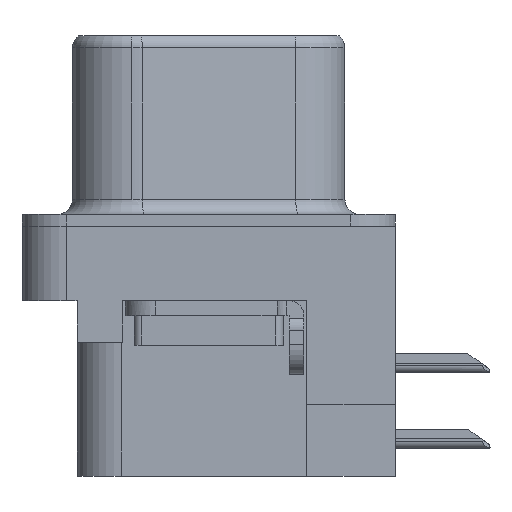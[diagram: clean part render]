
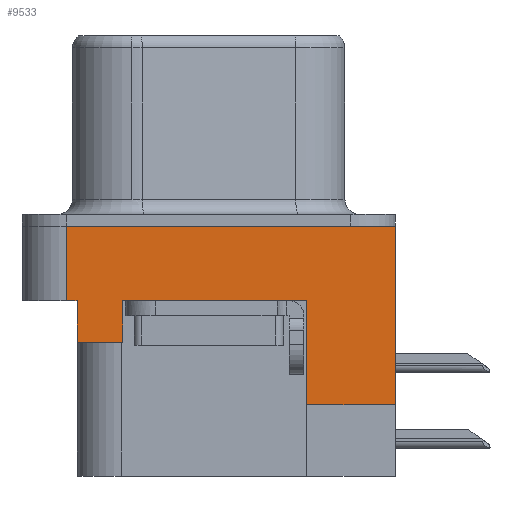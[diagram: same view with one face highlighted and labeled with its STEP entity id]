
A CAD part, left-side view. The second image highlights one B-rep face of the part: STEP entity #9533.
In plain terms, the highlighted planar face has unit normal (-1, 0, 0).
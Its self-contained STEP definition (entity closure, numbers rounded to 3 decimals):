
#211 = ORIENTED_EDGE ( 'NONE', *, *, #20539, .F. ) ;
#467 = VERTEX_POINT ( 'NONE', #12002 ) ;
#637 = VECTOR ( 'NONE', #18325, 1000. ) ;
#644 = CARTESIAN_POINT ( 'NONE',  ( -3., 2.895, -3.9 ) ) ;
#812 = LINE ( 'NONE', #14703, #637 ) ;
#1018 = DIRECTION ( 'NONE',  ( 0., 1., 0. ) ) ;
#1328 = AXIS2_PLACEMENT_3D ( 'NONE', #19992, #2776, #14723 ) ;
#1595 = ORIENTED_EDGE ( 'NONE', *, *, #21000, .T. ) ;
#1665 = DIRECTION ( 'NONE',  ( 0., 0., 1. ) ) ;
#2381 = VERTEX_POINT ( 'NONE', #3342 ) ;
#2776 = DIRECTION ( 'NONE',  ( -1., 0., 0. ) ) ;
#3298 = CARTESIAN_POINT ( 'NONE',  ( -3., 4.425, -3.9 ) ) ;
#3342 = CARTESIAN_POINT ( 'NONE',  ( -3., -3.295, -6. ) ) ;
#3749 = CARTESIAN_POINT ( 'NONE',  ( -3., -3.295, -2.5 ) ) ;
#4221 = ORIENTED_EDGE ( 'NONE', *, *, #19457, .T. ) ;
#5116 = VERTEX_POINT ( 'NONE', #3749 ) ;
#6253 = CARTESIAN_POINT ( 'NONE',  ( -3., -6.275, -2.5 ) ) ;
#7795 = EDGE_LOOP ( 'NONE', ( #10793, #1595, #10123, #9970, #10762, #18517, #211, #17232, #4221, #16567 ) ) ;
#8394 = DIRECTION ( 'NONE',  ( 0., 0., 1. ) ) ;
#9133 = VERTEX_POINT ( 'NONE', #22170 ) ;
#9533 = ADVANCED_FACE ( 'NONE', ( #13169 ), #16417, .T. ) ;
#9843 = DIRECTION ( 'NONE',  ( 0., 0., 1. ) ) ;
#9970 = ORIENTED_EDGE ( 'NONE', *, *, #21142, .F. ) ;
#10079 = CARTESIAN_POINT ( 'NONE',  ( -3., -6.275, 0. ) ) ;
#10123 = ORIENTED_EDGE ( 'NONE', *, *, #21007, .F. ) ;
#10279 = DIRECTION ( 'NONE',  ( 0., 1., 0. ) ) ;
#10762 = ORIENTED_EDGE ( 'NONE', *, *, #20664, .T. ) ;
#10793 = ORIENTED_EDGE ( 'NONE', *, *, #20972, .F. ) ;
#10803 = CARTESIAN_POINT ( 'NONE',  ( -3., 4.425, -3.9 ) ) ;
#11630 = VERTEX_POINT ( 'NONE', #10079 ) ;
#12002 = CARTESIAN_POINT ( 'NONE',  ( -3., -6.275, -6. ) ) ;
#12343 = DIRECTION ( 'NONE',  ( 0., -1., 0. ) ) ;
#12876 = VERTEX_POINT ( 'NONE', #17078 ) ;
#13169 = FACE_OUTER_BOUND ( 'NONE', #7795, .T. ) ;
#13196 = VERTEX_POINT ( 'NONE', #644 ) ;
#13553 = DIRECTION ( 'NONE',  ( 0., 0., 1. ) ) ;
#13590 = CARTESIAN_POINT ( 'NONE',  ( -3., 2.895, -3.9 ) ) ;
#13624 = CARTESIAN_POINT ( 'NONE',  ( -3., -3.295, -8.4 ) ) ;
#14703 = CARTESIAN_POINT ( 'NONE',  ( -3., -6.275, -2.5 ) ) ;
#14723 = DIRECTION ( 'NONE',  ( 0., 0., 1. ) ) ;
#14809 = CARTESIAN_POINT ( 'NONE',  ( -3., -6.275, 0. ) ) ;
#15319 = CARTESIAN_POINT ( 'NONE',  ( -3., 4.425, -2.5 ) ) ;
#15979 = VERTEX_POINT ( 'NONE', #19060 ) ;
#16347 = CARTESIAN_POINT ( 'NONE',  ( -3., -6.495, -6. ) ) ;
#16417 = PLANE ( 'NONE',  #1328 ) ;
#16511 = DIRECTION ( 'NONE',  ( 0., 0., 1. ) ) ;
#16567 = ORIENTED_EDGE ( 'NONE', *, *, #21261, .F. ) ;
#16581 = DIRECTION ( 'NONE',  ( 0., -1., 0. ) ) ;
#17078 = CARTESIAN_POINT ( 'NONE',  ( -3., 4.775, 0. ) ) ;
#17232 = ORIENTED_EDGE ( 'NONE', *, *, #19751, .T. ) ;
#17438 = LINE ( 'NONE', #13624, #17522 ) ;
#17477 = CARTESIAN_POINT ( 'NONE',  ( -3., -6.275, -2.5 ) ) ;
#17522 = VECTOR ( 'NONE', #1665, 1000. ) ;
#17549 = VECTOR ( 'NONE', #13553, 1000. ) ;
#17687 = LINE ( 'NONE', #3298, #17549 ) ;
#17759 = VECTOR ( 'NONE', #9843, 1000. ) ;
#17887 = LINE ( 'NONE', #18663, #17759 ) ;
#18215 = VECTOR ( 'NONE', #16581, 1000. ) ;
#18245 = VECTOR ( 'NONE', #16511, 1000. ) ;
#18263 = LINE ( 'NONE', #14809, #18215 ) ;
#18266 = LINE ( 'NONE', #6253, #18245 ) ;
#18325 = DIRECTION ( 'NONE',  ( 0., -1., 0. ) ) ;
#18430 = VECTOR ( 'NONE', #1018, 1000. ) ;
#18517 = ORIENTED_EDGE ( 'NONE', *, *, #21237, .F. ) ;
#18615 = LINE ( 'NONE', #16347, #18430 ) ;
#18663 = CARTESIAN_POINT ( 'NONE',  ( -3., 4.775, -2.5 ) ) ;
#19060 = CARTESIAN_POINT ( 'NONE',  ( -3., 4.775, -2.5 ) ) ;
#19224 = VERTEX_POINT ( 'NONE', #10803 ) ;
#19353 = VECTOR ( 'NONE', #12343, 1000. ) ;
#19457 = EDGE_CURVE ( 'NONE', #9133, #5116, #812, .T. ) ;
#19527 = LINE ( 'NONE', #17477, #19353 ) ;
#19712 = VECTOR ( 'NONE', #10279, 1000. ) ;
#19751 = EDGE_CURVE ( 'NONE', #13196, #9133, #21974, .T. ) ;
#19827 = LINE ( 'NONE', #20788, #19712 ) ;
#19992 = CARTESIAN_POINT ( 'NONE',  ( -3., -6.275, -2.5 ) ) ;
#20539 = EDGE_CURVE ( 'NONE', #13196, #19224, #19827, .T. ) ;
#20664 = EDGE_CURVE ( 'NONE', #15979, #21262, #19527, .T. ) ;
#20788 = CARTESIAN_POINT ( 'NONE',  ( -3., 4.425, -3.9 ) ) ;
#20972 = EDGE_CURVE ( 'NONE', #467, #2381, #18615, .T. ) ;
#21000 = EDGE_CURVE ( 'NONE', #467, #11630, #18266, .T. ) ;
#21007 = EDGE_CURVE ( 'NONE', #12876, #11630, #18263, .T. ) ;
#21142 = EDGE_CURVE ( 'NONE', #15979, #12876, #17887, .T. ) ;
#21237 = EDGE_CURVE ( 'NONE', #19224, #21262, #17687, .T. ) ;
#21261 = EDGE_CURVE ( 'NONE', #2381, #5116, #17438, .T. ) ;
#21262 = VERTEX_POINT ( 'NONE', #15319 ) ;
#21931 = VECTOR ( 'NONE', #8394, 1000. ) ;
#21974 = LINE ( 'NONE', #13590, #21931 ) ;
#22170 = CARTESIAN_POINT ( 'NONE',  ( -3., 2.895, -2.5 ) ) ;
